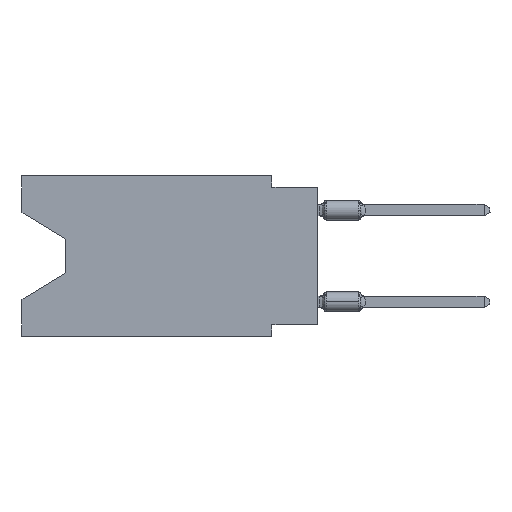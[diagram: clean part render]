
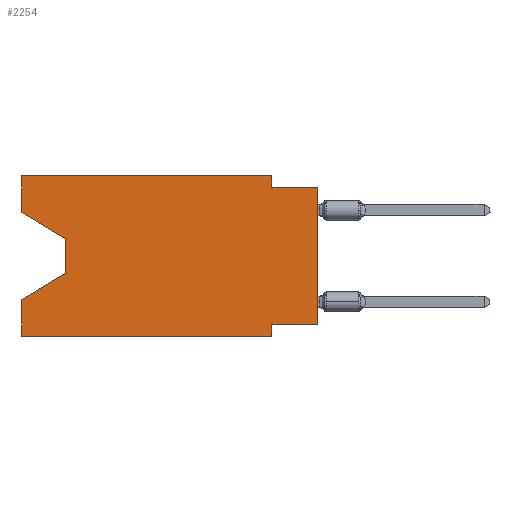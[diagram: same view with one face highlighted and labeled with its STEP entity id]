
A CAD part, left-side view. The second image highlights one B-rep face of the part: STEP entity #2254.
In plain terms, the highlighted planar face has unit normal (-1, 0, 0).
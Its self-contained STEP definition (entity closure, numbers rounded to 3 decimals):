
#69 = ORIENTED_EDGE ( 'NONE', *, *, #47185, .T. ) ;
#71 = DIRECTION ( 'NONE',  ( 0., -1., 0. ) ) ;
#1096 = CARTESIAN_POINT ( 'NONE',  ( 0., 2.54, -8.89 ) ) ;
#1535 = PLANE ( 'NONE',  #44345 ) ;
#1667 = VECTOR ( 'NONE', #12198, 1000. ) ;
#1706 = CARTESIAN_POINT ( 'NONE',  ( 0., 16.383, -8.89 ) ) ;
#1785 = ORIENTED_EDGE ( 'NONE', *, *, #41636, .T. ) ;
#1943 = LINE ( 'NONE', #42112, #11738 ) ;
#2254 = ADVANCED_FACE ( 'NONE', ( #45794 ), #1535, .F. ) ;
#2827 = VECTOR ( 'NONE', #9539, 1000. ) ;
#3517 = VECTOR ( 'NONE', #37992, 1000. ) ;
#3529 = CARTESIAN_POINT ( 'NONE',  ( 0., 16.383, 0. ) ) ;
#3771 = EDGE_CURVE ( 'NONE', #18581, #9021, #33264, .T. ) ;
#4031 = LINE ( 'NONE', #3529, #24691 ) ;
#4266 = EDGE_CURVE ( 'NONE', #30481, #5193, #46732, .T. ) ;
#5193 = VERTEX_POINT ( 'NONE', #44426 ) ;
#5319 = VECTOR ( 'NONE', #27049, 1000. ) ;
#5690 = CARTESIAN_POINT ( 'NONE',  ( 0., 16.383, -8.89 ) ) ;
#6612 = EDGE_CURVE ( 'NONE', #9027, #18581, #41780, .T. ) ;
#6871 = VECTOR ( 'NONE', #30264, 1000. ) ;
#8197 = LINE ( 'NONE', #31265, #3517 ) ;
#8542 = LINE ( 'NONE', #40772, #23215 ) ;
#9021 = VERTEX_POINT ( 'NONE', #11895 ) ;
#9027 = VERTEX_POINT ( 'NONE', #15265 ) ;
#9139 = LINE ( 'NONE', #19960, #41416 ) ;
#9168 = DIRECTION ( 'NONE',  ( 0., 0.855, -0.519 ) ) ;
#9278 = EDGE_CURVE ( 'NONE', #30165, #41379, #30648, .T. ) ;
#9539 = DIRECTION ( 'NONE',  ( 0., -1., 0. ) ) ;
#9599 = CARTESIAN_POINT ( 'NONE',  ( 0., 2.54, -0.635 ) ) ;
#10212 = ORIENTED_EDGE ( 'NONE', *, *, #6612, .F. ) ;
#11314 = VERTEX_POINT ( 'NONE', #24001 ) ;
#11670 = VERTEX_POINT ( 'NONE', #1096 ) ;
#11738 = VECTOR ( 'NONE', #9168, 1000. ) ;
#11895 = CARTESIAN_POINT ( 'NONE',  ( 0., 0., -0.635 ) ) ;
#12198 = DIRECTION ( 'NONE',  ( 0., 0., -1. ) ) ;
#12349 = CARTESIAN_POINT ( 'NONE',  ( 0., 16.383, -6.852 ) ) ;
#12456 = LINE ( 'NONE', #23047, #6871 ) ;
#15265 = CARTESIAN_POINT ( 'NONE',  ( 0., 2.54, 0. ) ) ;
#15483 = ORIENTED_EDGE ( 'NONE', *, *, #46788, .F. ) ;
#15753 = ORIENTED_EDGE ( 'NONE', *, *, #4266, .T. ) ;
#15979 = ORIENTED_EDGE ( 'NONE', *, *, #9278, .F. ) ;
#16746 = LINE ( 'NONE', #5690, #2827 ) ;
#17704 = ORIENTED_EDGE ( 'NONE', *, *, #19153, .F. ) ;
#18101 = CARTESIAN_POINT ( 'NONE',  ( 0., 13.97, -3.505 ) ) ;
#18581 = VERTEX_POINT ( 'NONE', #9599 ) ;
#19153 = EDGE_CURVE ( 'NONE', #11314, #9027, #8542, .T. ) ;
#19360 = DIRECTION ( 'NONE',  ( 0., -1., 0. ) ) ;
#19631 = EDGE_CURVE ( 'NONE', #5193, #42448, #1943, .T. ) ;
#19960 = CARTESIAN_POINT ( 'NONE',  ( 0., 16.383, 0. ) ) ;
#20065 = DIRECTION ( 'NONE',  ( 1., 0., 0. ) ) ;
#22300 = VERTEX_POINT ( 'NONE', #1706 ) ;
#22356 = CARTESIAN_POINT ( 'NONE',  ( 0., 13.97, -3.505 ) ) ;
#22872 = CARTESIAN_POINT ( 'NONE',  ( 0., 2.54, -8.89 ) ) ;
#22913 = CARTESIAN_POINT ( 'NONE',  ( 0., 0., -0.635 ) ) ;
#23047 = CARTESIAN_POINT ( 'NONE',  ( 0., 16.383, -2.038 ) ) ;
#23215 = VECTOR ( 'NONE', #19360, 1000. ) ;
#24001 = CARTESIAN_POINT ( 'NONE',  ( 0., 16.383, 0. ) ) ;
#24691 = VECTOR ( 'NONE', #25429, 1000. ) ;
#25429 = DIRECTION ( 'NONE',  ( 0., 0., 1. ) ) ;
#26120 = VECTOR ( 'NONE', #28917, 1000. ) ;
#26830 = VECTOR ( 'NONE', #71, 1000. ) ;
#27049 = DIRECTION ( 'NONE',  ( 0., 1., 0. ) ) ;
#27122 = VERTEX_POINT ( 'NONE', #39265 ) ;
#27277 = DIRECTION ( 'NONE',  ( 0., 0., -1. ) ) ;
#27281 = CARTESIAN_POINT ( 'NONE',  ( 0., 0., -8.255 ) ) ;
#28917 = DIRECTION ( 'NONE',  ( 0., 0., -1. ) ) ;
#29189 = ORIENTED_EDGE ( 'NONE', *, *, #41638, .F. ) ;
#30165 = VERTEX_POINT ( 'NONE', #38720 ) ;
#30264 = DIRECTION ( 'NONE',  ( 0., -0.855, -0.519 ) ) ;
#30481 = VERTEX_POINT ( 'NONE', #22356 ) ;
#30607 = ORIENTED_EDGE ( 'NONE', *, *, #3771, .F. ) ;
#30648 = LINE ( 'NONE', #27281, #5319 ) ;
#30832 = EDGE_CURVE ( 'NONE', #22300, #42448, #4031, .T. ) ;
#31265 = CARTESIAN_POINT ( 'NONE',  ( 0., 0., 0. ) ) ;
#31273 = EDGE_LOOP ( 'NONE', ( #69, #15753, #33414, #44973, #46441, #29189, #15979, #1785, #30607, #10212, #17704, #15483 ) ) ;
#33264 = LINE ( 'NONE', #22913, #26830 ) ;
#33414 = ORIENTED_EDGE ( 'NONE', *, *, #19631, .T. ) ;
#34151 = DIRECTION ( 'NONE',  ( 0., 0., -1. ) ) ;
#35030 = CARTESIAN_POINT ( 'NONE',  ( 0., 2.54, 0. ) ) ;
#37992 = DIRECTION ( 'NONE',  ( 0., 0., 1. ) ) ;
#38474 = LINE ( 'NONE', #22872, #43466 ) ;
#38566 = CARTESIAN_POINT ( 'NONE',  ( 0., 16.383, 0. ) ) ;
#38720 = CARTESIAN_POINT ( 'NONE',  ( 0., 0., -8.255 ) ) ;
#39265 = CARTESIAN_POINT ( 'NONE',  ( 0., 16.383, -2.038 ) ) ;
#40772 = CARTESIAN_POINT ( 'NONE',  ( 0., 16.383, 0. ) ) ;
#41379 = VERTEX_POINT ( 'NONE', #46700 ) ;
#41416 = VECTOR ( 'NONE', #42084, 1000. ) ;
#41636 = EDGE_CURVE ( 'NONE', #30165, #9021, #8197, .T. ) ;
#41638 = EDGE_CURVE ( 'NONE', #41379, #11670, #38474, .T. ) ;
#41780 = LINE ( 'NONE', #35030, #1667 ) ;
#42084 = DIRECTION ( 'NONE',  ( 0., 0., 1. ) ) ;
#42112 = CARTESIAN_POINT ( 'NONE',  ( 0., 13.97, -5.385 ) ) ;
#42448 = VERTEX_POINT ( 'NONE', #12349 ) ;
#43466 = VECTOR ( 'NONE', #34151, 1000. ) ;
#44345 = AXIS2_PLACEMENT_3D ( 'NONE', #38566, #20065, #27277 ) ;
#44383 = EDGE_CURVE ( 'NONE', #22300, #11670, #16746, .T. ) ;
#44426 = CARTESIAN_POINT ( 'NONE',  ( 0., 13.97, -5.385 ) ) ;
#44973 = ORIENTED_EDGE ( 'NONE', *, *, #30832, .F. ) ;
#45794 = FACE_OUTER_BOUND ( 'NONE', #31273, .T. ) ;
#46441 = ORIENTED_EDGE ( 'NONE', *, *, #44383, .T. ) ;
#46700 = CARTESIAN_POINT ( 'NONE',  ( 0., 2.54, -8.255 ) ) ;
#46732 = LINE ( 'NONE', #18101, #26120 ) ;
#46788 = EDGE_CURVE ( 'NONE', #27122, #11314, #9139, .T. ) ;
#47185 = EDGE_CURVE ( 'NONE', #27122, #30481, #12456, .T. ) ;
